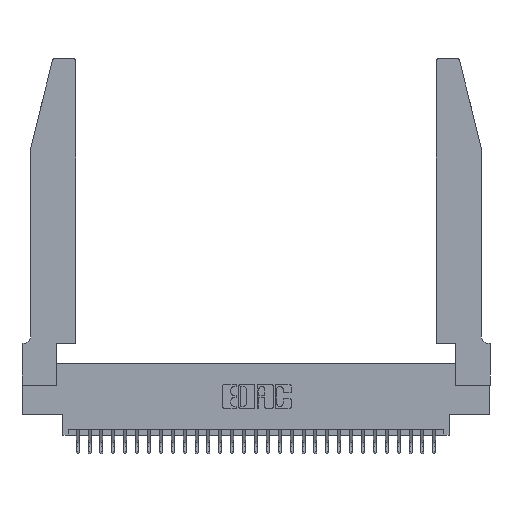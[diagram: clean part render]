
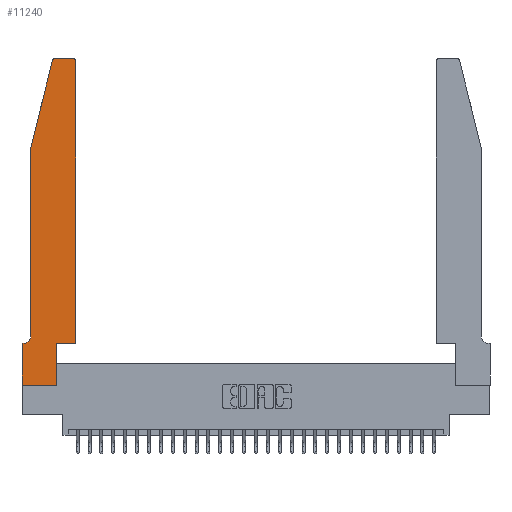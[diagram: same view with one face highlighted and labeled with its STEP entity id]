
A CAD part, top view. The second image highlights one B-rep face of the part: STEP entity #11240.
In plain terms, the highlighted planar face has unit normal (0, 0, 1).
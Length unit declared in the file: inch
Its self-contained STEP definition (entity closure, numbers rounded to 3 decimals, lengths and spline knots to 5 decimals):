
#385 = CARTESIAN_POINT ( 'NONE',  ( 0.4505, 0.35, 0.37 ) ) ;
#552 = AXIS2_PLACEMENT_3D ( 'NONE', #26878, #29293, #3214 ) ;
#618 = ORIENTED_EDGE ( 'NONE', *, *, #15811, .T. ) ;
#692 = ORIENTED_EDGE ( 'NONE', *, *, #13525, .T. ) ;
#1746 = PLANE ( 'NONE',  #13278 ) ;
#1813 = AXIS2_PLACEMENT_3D ( 'NONE', #14594, #24339, #11967 ) ;
#2768 = VECTOR ( 'NONE', #25975, 39.37008 ) ;
#2936 = VERTEX_POINT ( 'NONE', #385 ) ;
#3214 = DIRECTION ( 'NONE',  ( 1., 0., 0. ) ) ;
#3859 = LINE ( 'NONE', #17822, #28507 ) ;
#4180 = LINE ( 'NONE', #30643, #29551 ) ;
#4479 = ORIENTED_EDGE ( 'NONE', *, *, #29522, .T. ) ;
#5192 = LINE ( 'NONE', #19073, #12321 ) ;
#5249 = VERTEX_POINT ( 'NONE', #20995 ) ;
#5927 = ORIENTED_EDGE ( 'NONE', *, *, #19346, .T. ) ;
#6475 = LINE ( 'NONE', #23583, #14741 ) ;
#6595 = CARTESIAN_POINT ( 'NONE',  ( 0.2865, 0.35, 0.37 ) ) ;
#6708 = CIRCLE ( 'NONE', #552, 0.03 ) ;
#6748 = DIRECTION ( 'NONE',  ( -1., 0., 0. ) ) ;
#7288 = VERTEX_POINT ( 'NONE', #17434 ) ;
#7382 = EDGE_CURVE ( 'NONE', #5249, #15397, #6708, .T. ) ;
#7899 = CARTESIAN_POINT ( 'NONE',  ( 0.4205, 2.75, 0.37 ) ) ;
#8275 = VECTOR ( 'NONE', #30465, 39.37008 ) ;
#8376 = LINE ( 'NONE', #17231, #2768 ) ;
#9064 = VECTOR ( 'NONE', #21051, 39.37008 ) ;
#9075 = EDGE_CURVE ( 'NONE', #7288, #22545, #24494, .T. ) ;
#9850 = CARTESIAN_POINT ( 'NONE',  ( 0.4505, 2.72, 0.37 ) ) ;
#11240 = ADVANCED_FACE ( 'NONE', ( #27001 ), #1746, .T. ) ;
#11383 = DIRECTION ( 'NONE',  ( 0., 0., 1. ) ) ;
#11660 = LINE ( 'NONE', #30573, #8275 ) ;
#11855 = ORIENTED_EDGE ( 'NONE', *, *, #23793, .T. ) ;
#11883 = VERTEX_POINT ( 'NONE', #6595 ) ;
#11967 = DIRECTION ( 'NONE',  ( 1., 0., 0. ) ) ;
#11973 = VERTEX_POINT ( 'NONE', #30490 ) ;
#12321 = VECTOR ( 'NONE', #28460, 39.37008 ) ;
#12442 = EDGE_CURVE ( 'NONE', #15397, #22386, #11660, .T. ) ;
#13278 = AXIS2_PLACEMENT_3D ( 'NONE', #25736, #11383, #20842 ) ;
#13356 = VERTEX_POINT ( 'NONE', #7899 ) ;
#13525 = EDGE_CURVE ( 'NONE', #22386, #14284, #20328, .T. ) ;
#14093 = CARTESIAN_POINT ( 'NONE',  ( 0.0755, 2., 0.37 ) ) ;
#14284 = VERTEX_POINT ( 'NONE', #26518 ) ;
#14594 = CARTESIAN_POINT ( 'NONE',  ( 0.4205, 2.72, 0.37 ) ) ;
#14741 = VECTOR ( 'NONE', #23165, 39.37008 ) ;
#15397 = VERTEX_POINT ( 'NONE', #26876 ) ;
#15811 = EDGE_CURVE ( 'NONE', #21279, #11973, #4180, .T. ) ;
#15869 = DIRECTION ( 'NONE',  ( 0., 0., -1. ) ) ;
#16015 = VERTEX_POINT ( 'NONE', #9850 ) ;
#16166 = DIRECTION ( 'NONE',  ( 0., -1., 0. ) ) ;
#16286 = VECTOR ( 'NONE', #16166, 39.37008 ) ;
#16403 = CARTESIAN_POINT ( 'NONE',  ( 0.0755, 2., 0.37 ) ) ;
#16518 = CARTESIAN_POINT ( 'NONE',  ( 0.4505, 0.35, 0.37 ) ) ;
#17231 = CARTESIAN_POINT ( 'NONE',  ( 0.2865, 0.35, 0.37 ) ) ;
#17249 = CIRCLE ( 'NONE', #29013, 0.07 ) ;
#17434 = CARTESIAN_POINT ( 'NONE',  ( 0., 0., 0.37 ) ) ;
#17822 = CARTESIAN_POINT ( 'NONE',  ( 0.4505, 0.35, 0.37 ) ) ;
#17927 = DIRECTION ( 'NONE',  ( 1., 0., 0. ) ) ;
#18121 = ORIENTED_EDGE ( 'NONE', *, *, #28943, .T. ) ;
#18839 = ORIENTED_EDGE ( 'NONE', *, *, #26021, .T. ) ;
#19073 = CARTESIAN_POINT ( 'NONE',  ( 0., 0., 0.37 ) ) ;
#19346 = EDGE_CURVE ( 'NONE', #22545, #11883, #8376, .T. ) ;
#19462 = CARTESIAN_POINT ( 'NONE',  ( 0.2865, 0., 0.37 ) ) ;
#19721 = ORIENTED_EDGE ( 'NONE', *, *, #7382, .T. ) ;
#19875 = CARTESIAN_POINT ( 'NONE',  ( 0.0055, 0.35, 0.37 ) ) ;
#20328 = LINE ( 'NONE', #14093, #16286 ) ;
#20412 = CARTESIAN_POINT ( 'NONE',  ( 0.0055, 0.42, 0.37 ) ) ;
#20842 = DIRECTION ( 'NONE',  ( 1., 0., 0. ) ) ;
#20989 = LINE ( 'NONE', #16518, #9064 ) ;
#20995 = CARTESIAN_POINT ( 'NONE',  ( 0.284, 2.75, 0.37 ) ) ;
#21051 = DIRECTION ( 'NONE',  ( 0., 1., 0. ) ) ;
#21279 = VERTEX_POINT ( 'NONE', #19875 ) ;
#22386 = VERTEX_POINT ( 'NONE', #16403 ) ;
#22466 = EDGE_CURVE ( 'NONE', #16015, #13356, #22515, .T. ) ;
#22515 = CIRCLE ( 'NONE', #1813, 0.03 ) ;
#22545 = VERTEX_POINT ( 'NONE', #19462 ) ;
#22804 = EDGE_CURVE ( 'NONE', #11883, #2936, #3859, .T. ) ;
#23165 = DIRECTION ( 'NONE',  ( -1., 0., 0. ) ) ;
#23583 = CARTESIAN_POINT ( 'NONE',  ( 0.2605, 2.75, 0.37 ) ) ;
#23593 = EDGE_LOOP ( 'NONE', ( #18121, #19721, #28625, #692, #11855, #618, #18839, #25988, #5927, #28901, #4479, #24738 ) ) ;
#23793 = EDGE_CURVE ( 'NONE', #14284, #21279, #17249, .T. ) ;
#24339 = DIRECTION ( 'NONE',  ( 0., 0., 1. ) ) ;
#24494 = LINE ( 'NONE', #27322, #29726 ) ;
#24738 = ORIENTED_EDGE ( 'NONE', *, *, #22466, .T. ) ;
#25024 = DIRECTION ( 'NONE',  ( 1., 0., 0. ) ) ;
#25736 = CARTESIAN_POINT ( 'NONE',  ( 0., 0.35, 0.37 ) ) ;
#25975 = DIRECTION ( 'NONE',  ( 0., 1., 0. ) ) ;
#25988 = ORIENTED_EDGE ( 'NONE', *, *, #9075, .T. ) ;
#26021 = EDGE_CURVE ( 'NONE', #11973, #7288, #5192, .T. ) ;
#26518 = CARTESIAN_POINT ( 'NONE',  ( 0.0755, 0.42, 0.37 ) ) ;
#26876 = CARTESIAN_POINT ( 'NONE',  ( 0.25487, 2.72718, 0.37 ) ) ;
#26878 = CARTESIAN_POINT ( 'NONE',  ( 0.284, 2.72, 0.37 ) ) ;
#27001 = FACE_OUTER_BOUND ( 'NONE', #23593, .T. ) ;
#27322 = CARTESIAN_POINT ( 'NONE',  ( 0., 0., 0.37 ) ) ;
#28460 = DIRECTION ( 'NONE',  ( 0., -1., 0. ) ) ;
#28507 = VECTOR ( 'NONE', #17927, 39.37008 ) ;
#28625 = ORIENTED_EDGE ( 'NONE', *, *, #12442, .T. ) ;
#28901 = ORIENTED_EDGE ( 'NONE', *, *, #22804, .T. ) ;
#28943 = EDGE_CURVE ( 'NONE', #13356, #5249, #6475, .T. ) ;
#29013 = AXIS2_PLACEMENT_3D ( 'NONE', #20412, #15869, #30317 ) ;
#29293 = DIRECTION ( 'NONE',  ( 0., 0., 1. ) ) ;
#29522 = EDGE_CURVE ( 'NONE', #2936, #16015, #20989, .T. ) ;
#29551 = VECTOR ( 'NONE', #6748, 39.37008 ) ;
#29726 = VECTOR ( 'NONE', #25024, 39.37008 ) ;
#30317 = DIRECTION ( 'NONE',  ( -1., 0., 0. ) ) ;
#30465 = DIRECTION ( 'NONE',  ( -0.239, -0.971, 0. ) ) ;
#30490 = CARTESIAN_POINT ( 'NONE',  ( 0., 0.35, 0.37 ) ) ;
#30573 = CARTESIAN_POINT ( 'NONE',  ( 0.0755, 2., 0.37 ) ) ;
#30643 = CARTESIAN_POINT ( 'NONE',  ( 0.0755, 0.35, 0.37 ) ) ;
